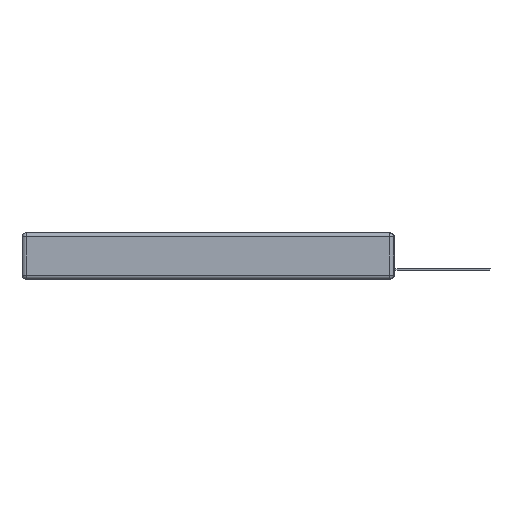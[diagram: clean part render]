
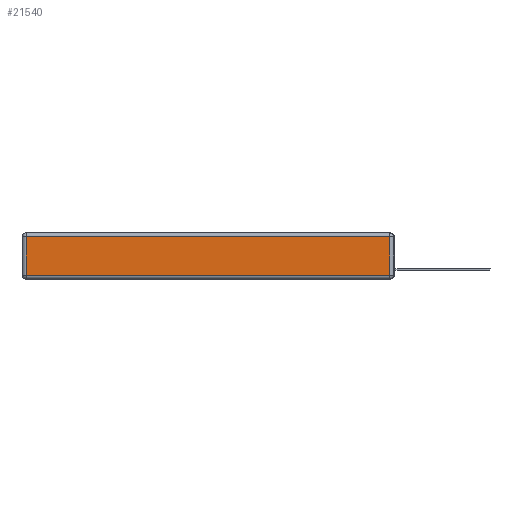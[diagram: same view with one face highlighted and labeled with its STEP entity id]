
A CAD part, left-side view. The second image highlights one B-rep face of the part: STEP entity #21540.
In plain terms, the highlighted planar face has unit normal (-1, 0, 0).
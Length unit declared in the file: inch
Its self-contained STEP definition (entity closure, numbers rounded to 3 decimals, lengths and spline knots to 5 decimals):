
#396 = VECTOR ( 'NONE', #7896, 39.37008 ) ;
#948 = CARTESIAN_POINT ( 'NONE',  ( 0., 2.75, -0.03 ) ) ;
#1698 = VERTEX_POINT ( 'NONE', #18619 ) ;
#1883 = DIRECTION ( 'NONE',  ( 0., 0., 1. ) ) ;
#2398 = CARTESIAN_POINT ( 'NONE',  ( 0., 2.72, -0.313 ) ) ;
#2596 = FACE_OUTER_BOUND ( 'NONE', #24534, .T. ) ;
#3968 = CARTESIAN_POINT ( 'NONE',  ( 0., 0., -0.313 ) ) ;
#4219 = LINE ( 'NONE', #13606, #10989 ) ;
#5398 = VECTOR ( 'NONE', #6559, 39.37008 ) ;
#6029 = ORIENTED_EDGE ( 'NONE', *, *, #15584, .T. ) ;
#6285 = DIRECTION ( 'NONE',  ( 0., 0., 1. ) ) ;
#6512 = VERTEX_POINT ( 'NONE', #2398 ) ;
#6559 = DIRECTION ( 'NONE',  ( 0., 1., 0. ) ) ;
#6742 = LINE ( 'NONE', #8570, #16904 ) ;
#6946 = LINE ( 'NONE', #948, #5398 ) ;
#7434 = EDGE_CURVE ( 'NONE', #6512, #16415, #15497, .T. ) ;
#7896 = DIRECTION ( 'NONE',  ( 0., -1., 0. ) ) ;
#8570 = CARTESIAN_POINT ( 'NONE',  ( 0., 2.72, -0.343 ) ) ;
#9803 = EDGE_CURVE ( 'NONE', #20828, #6512, #6742, .T. ) ;
#10357 = DIRECTION ( 'NONE',  ( -1., 0., 0. ) ) ;
#10989 = VECTOR ( 'NONE', #1883, 39.37008 ) ;
#11741 = ORIENTED_EDGE ( 'NONE', *, *, #20985, .T. ) ;
#13606 = CARTESIAN_POINT ( 'NONE',  ( 0., 0.03, -0.343 ) ) ;
#14721 = ORIENTED_EDGE ( 'NONE', *, *, #9803, .T. ) ;
#15497 = LINE ( 'NONE', #3968, #396 ) ;
#15584 = EDGE_CURVE ( 'NONE', #16415, #1698, #4219, .T. ) ;
#16415 = VERTEX_POINT ( 'NONE', #25404 ) ;
#16904 = VECTOR ( 'NONE', #22432, 39.37008 ) ;
#18013 = CARTESIAN_POINT ( 'NONE',  ( 0., 2.72, -0.03 ) ) ;
#18619 = CARTESIAN_POINT ( 'NONE',  ( 0., 0.03, -0.03 ) ) ;
#20828 = VERTEX_POINT ( 'NONE', #18013 ) ;
#20985 = EDGE_CURVE ( 'NONE', #1698, #20828, #6946, .T. ) ;
#21540 = ADVANCED_FACE ( 'NONE', ( #2596 ), #22124, .T. ) ;
#21706 = AXIS2_PLACEMENT_3D ( 'NONE', #23945, #10357, #6285 ) ;
#22124 = PLANE ( 'NONE',  #21706 ) ;
#22432 = DIRECTION ( 'NONE',  ( 0., 0., -1. ) ) ;
#23662 = ORIENTED_EDGE ( 'NONE', *, *, #7434, .T. ) ;
#23945 = CARTESIAN_POINT ( 'NONE',  ( 0., 0., -0.343 ) ) ;
#24534 = EDGE_LOOP ( 'NONE', ( #23662, #6029, #11741, #14721 ) ) ;
#25404 = CARTESIAN_POINT ( 'NONE',  ( 0., 0.03, -0.313 ) ) ;
